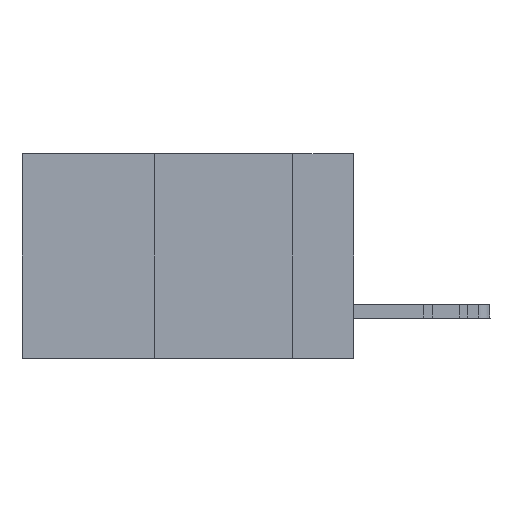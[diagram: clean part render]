
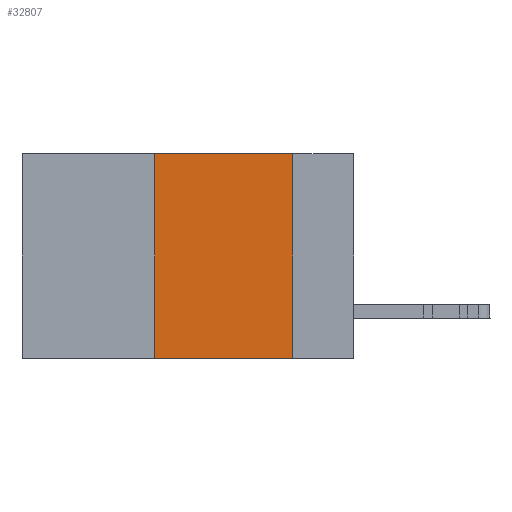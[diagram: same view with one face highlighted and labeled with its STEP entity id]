
A CAD part, left-side view. The second image highlights one B-rep face of the part: STEP entity #32807.
In plain terms, the highlighted planar face has unit normal (-1, 0, 0).
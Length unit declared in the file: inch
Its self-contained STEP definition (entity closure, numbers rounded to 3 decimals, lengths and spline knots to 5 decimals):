
#666 = CARTESIAN_POINT ( 'NONE',  ( 0., 0.11, 0. ) ) ;
#1776 = VERTEX_POINT ( 'NONE', #41887 ) ;
#2094 = CARTESIAN_POINT ( 'NONE',  ( 0., 0.6, -0.37 ) ) ;
#3970 = DIRECTION ( 'NONE',  ( 0., 0., -1. ) ) ;
#4827 = CARTESIAN_POINT ( 'NONE',  ( 0., 0.36, -0.37 ) ) ;
#5145 = VECTOR ( 'NONE', #7282, 39.37008 ) ;
#5531 = VECTOR ( 'NONE', #17090, 39.37008 ) ;
#6114 = ORIENTED_EDGE ( 'NONE', *, *, #6571, .F. ) ;
#6571 = EDGE_CURVE ( 'NONE', #43043, #34507, #25122, .T. ) ;
#7282 = DIRECTION ( 'NONE',  ( 0., -1., 0. ) ) ;
#11706 = LINE ( 'NONE', #666, #19564 ) ;
#12043 = CARTESIAN_POINT ( 'NONE',  ( 0., 0.6, 0. ) ) ;
#13322 = CARTESIAN_POINT ( 'NONE',  ( 0., 0.36, 0. ) ) ;
#13535 = LINE ( 'NONE', #28849, #5145 ) ;
#17090 = DIRECTION ( 'NONE',  ( 0., 0., 1. ) ) ;
#18415 = LINE ( 'NONE', #2094, #25638 ) ;
#19564 = VECTOR ( 'NONE', #3970, 39.37008 ) ;
#23797 = EDGE_CURVE ( 'NONE', #43043, #1776, #18415, .T. ) ;
#25122 = LINE ( 'NONE', #25254, #5531 ) ;
#25254 = CARTESIAN_POINT ( 'NONE',  ( 0., 0.36, 0. ) ) ;
#25414 = ORIENTED_EDGE ( 'NONE', *, *, #35220, .F. ) ;
#25638 = VECTOR ( 'NONE', #45224, 39.37008 ) ;
#28316 = ORIENTED_EDGE ( 'NONE', *, *, #36577, .F. ) ;
#28735 = VERTEX_POINT ( 'NONE', #32933 ) ;
#28849 = CARTESIAN_POINT ( 'NONE',  ( 0., 0.6, 0. ) ) ;
#29584 = PLANE ( 'NONE',  #45070 ) ;
#32807 = ADVANCED_FACE ( 'NONE', ( #43113 ), #29584, .F. ) ;
#32933 = CARTESIAN_POINT ( 'NONE',  ( 0., 0.11, 0. ) ) ;
#33224 = DIRECTION ( 'NONE',  ( 1., 0., 0. ) ) ;
#34507 = VERTEX_POINT ( 'NONE', #13322 ) ;
#35220 = EDGE_CURVE ( 'NONE', #34507, #28735, #13535, .T. ) ;
#36577 = EDGE_CURVE ( 'NONE', #28735, #1776, #11706, .T. ) ;
#39566 = EDGE_LOOP ( 'NONE', ( #28316, #25414, #6114, #39586 ) ) ;
#39586 = ORIENTED_EDGE ( 'NONE', *, *, #23797, .T. ) ;
#40634 = DIRECTION ( 'NONE',  ( 0., 0., -1. ) ) ;
#41887 = CARTESIAN_POINT ( 'NONE',  ( 0., 0.11, -0.37 ) ) ;
#43043 = VERTEX_POINT ( 'NONE', #4827 ) ;
#43113 = FACE_OUTER_BOUND ( 'NONE', #39566, .T. ) ;
#45070 = AXIS2_PLACEMENT_3D ( 'NONE', #12043, #33224, #40634 ) ;
#45224 = DIRECTION ( 'NONE',  ( 0., -1., 0. ) ) ;
